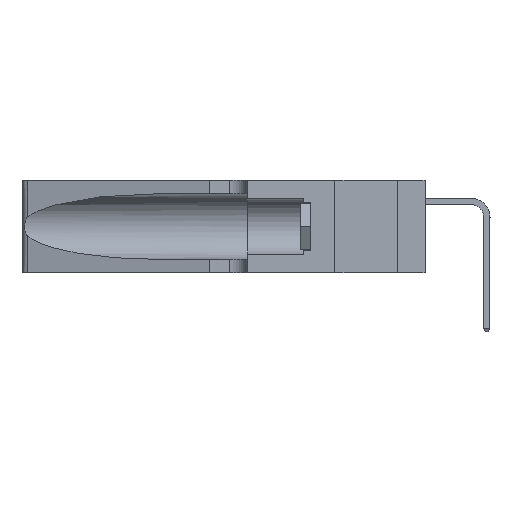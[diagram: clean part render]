
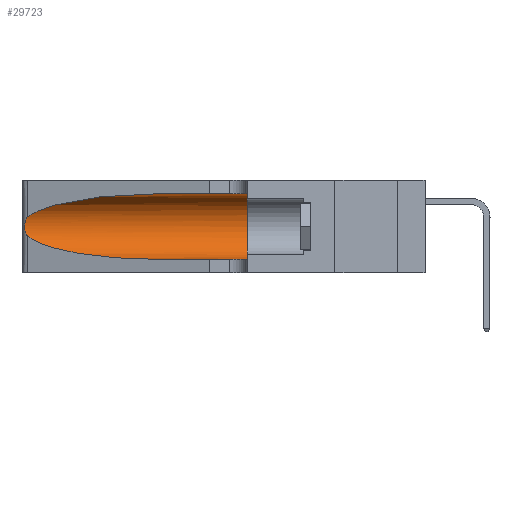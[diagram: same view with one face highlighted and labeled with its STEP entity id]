
A CAD part, left-side view. The second image highlights one B-rep face of the part: STEP entity #29723.
In plain terms, the highlighted cylindrical face has radius 3.308 mm (diameter 6.617 mm), a partial arc.
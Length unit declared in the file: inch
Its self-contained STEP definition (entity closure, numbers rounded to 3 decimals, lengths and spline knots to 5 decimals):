
#167 = ORIENTED_EDGE ( 'NONE', *, *, #20229, .T. ) ;
#437 = AXIS2_PLACEMENT_3D ( 'NONE', #23737, #39651, #20518 ) ;
#1509 = CARTESIAN_POINT ( 'NONE',  ( 0.25487, 1.22718, 0.22369 ) ) ;
#1642 = CARTESIAN_POINT ( 'NONE',  ( 0.25856, 1.23593, 0.16098 ) ) ;
#2059 = VERTEX_POINT ( 'NONE', #39702 ) ;
#2282 = VERTEX_POINT ( 'NONE', #24754 ) ;
#3160 = ORIENTED_EDGE ( 'NONE', *, *, #30647, .F. ) ;
#4863 = CARTESIAN_POINT ( 'NONE',  ( 0.25639, 1.23186, 0.15144 ) ) ;
#5967 = CARTESIAN_POINT ( 'NONE',  ( 0.18966, 0.96281, 0.31525 ) ) ;
#6445 = CARTESIAN_POINT ( 'NONE',  ( 0.25487, 1.22718, 0.14631 ) ) ;
#8058 = CARTESIAN_POINT ( 'NONE',  ( 0.25487, 1.22718, 0.14631 ) ) ;
#9328 = LINE ( 'NONE', #19906, #35790 ) ;
#9596 = CARTESIAN_POINT ( 'NONE',  ( 0.1305, 0.35, 0.05475 ) ) ;
#10426 = CYLINDRICAL_SURFACE ( 'NONE', #437, 0.13025 ) ;
#11134 = CARTESIAN_POINT ( 'NONE',  ( 0.25639, 1.23184, 0.21858 ) ) ;
#11966 = EDGE_CURVE ( 'NONE', #2282, #15474, #9328, .T. ) ;
#12347 = CARTESIAN_POINT ( 'NONE',  ( 0.1305, 1.61858, 0.31525 ) ) ;
#14373 = CARTESIAN_POINT ( 'NONE',  ( 0.25854, 1.2359, 0.20912 ) ) ;
#14772 = CARTESIAN_POINT ( 'NONE',  ( 0.1305, 0.35, 0.185 ) ) ;
#15474 = VERTEX_POINT ( 'NONE', #9596 ) ;
#15602 = CARTESIAN_POINT ( 'NONE',  ( 0.1305, 0.72297, 0.31525 ) ) ;
#15966 = AXIS2_PLACEMENT_3D ( 'NONE', #14772, #37096, #17969 ) ;
#16112 = CARTESIAN_POINT ( 'NONE',  ( 0.2373, 1.15595, 0.08982 ) ) ;
#16342 = CARTESIAN_POINT ( 'NONE',  ( 0.1305, 0.72297, 0.31525 ) ) ;
#16795 = VERTEX_POINT ( 'NONE', #16342 ) ;
#17569 = CARTESIAN_POINT ( 'NONE',  ( 0.26075, 1.23896, 0.19203 ) ) ;
#17969 = DIRECTION ( 'NONE',  ( 0., 0., 1. ) ) ;
#18198 =( BOUNDED_CURVE ( )  B_SPLINE_CURVE ( 3, ( #35230, #16112, #38451, #19336 ),
 .UNSPECIFIED., .F., .F. ) 
 B_SPLINE_CURVE_WITH_KNOTS ( ( 4, 4 ),
 ( 3.44316, 4.71239 ),
 .UNSPECIFIED. ) 
 CURVE ( )  GEOMETRIC_REPRESENTATION_ITEM ( )  RATIONAL_B_SPLINE_CURVE ( ( 1., 0.87, 0.87, 1. ) ) 
 REPRESENTATION_ITEM ( '' )  );
#18345 = VERTEX_POINT ( 'NONE', #6445 ) ;
#18705 = ORIENTED_EDGE ( 'NONE', *, *, #19258, .F. ) ;
#18824 = CARTESIAN_POINT ( 'NONE',  ( 0.2373, 1.15595, 0.28018 ) ) ;
#19258 = EDGE_CURVE ( 'NONE', #2059, #15474, #34302, .T. ) ;
#19336 = CARTESIAN_POINT ( 'NONE',  ( 0.1305, 0.72297, 0.05475 ) ) ;
#19906 = CARTESIAN_POINT ( 'NONE',  ( 0.1305, 1.61858, 0.05475 ) ) ;
#20229 = EDGE_CURVE ( 'NONE', #24245, #18345, #38668, .T. ) ;
#20293 = EDGE_LOOP ( 'NONE', ( #31163, #167, #30415, #21150, #18705, #3160 ) ) ;
#20518 = DIRECTION ( 'NONE',  ( 0., 0., -1. ) ) ;
#20784 = CARTESIAN_POINT ( 'NONE',  ( 0.26017, 1.23833, 0.17102 ) ) ;
#21100 = EDGE_CURVE ( 'NONE', #18345, #2282, #18198, .T. ) ;
#21150 = ORIENTED_EDGE ( 'NONE', *, *, #11966, .T. ) ;
#23116 = DIRECTION ( 'NONE',  ( 0., -1., 0. ) ) ;
#23737 = CARTESIAN_POINT ( 'NONE',  ( 0.1305, 1.61858, 0.185 ) ) ;
#24008 = CARTESIAN_POINT ( 'NONE',  ( 0.25789, 1.23486, 0.15765 ) ) ;
#24245 = VERTEX_POINT ( 'NONE', #39975 ) ;
#24754 = CARTESIAN_POINT ( 'NONE',  ( 0.1305, 0.72297, 0.05475 ) ) ;
#25411 =( BOUNDED_CURVE ( )  B_SPLINE_CURVE ( 3, ( #15602, #5967, #18824, #41153 ),
 .UNSPECIFIED., .F., .T. ) 
 B_SPLINE_CURVE_WITH_KNOTS ( ( 4, 4 ),
 ( 1.5708, 2.84003 ),
 .UNSPECIFIED. ) 
 CURVE ( )  GEOMETRIC_REPRESENTATION_ITEM ( )  RATIONAL_B_SPLINE_CURVE ( ( 1., 0.87, 0.87, 1. ) ) 
 REPRESENTATION_ITEM ( '' )  );
#27078 = CARTESIAN_POINT ( 'NONE',  ( 0.25555, 1.22994, 0.2215 ) ) ;
#27213 = CARTESIAN_POINT ( 'NONE',  ( 0.25555, 1.22993, 0.14849 ) ) ;
#27565 = EDGE_CURVE ( 'NONE', #16795, #24245, #25411, .T. ) ;
#29723 = ADVANCED_FACE ( 'NONE', ( #35887 ), #10426, .F. ) ;
#30415 = ORIENTED_EDGE ( 'NONE', *, *, #21100, .T. ) ;
#30647 = EDGE_CURVE ( 'NONE', #16795, #2059, #40603, .T. ) ;
#31163 = ORIENTED_EDGE ( 'NONE', *, *, #27565, .T. ) ;
#33114 = VECTOR ( 'NONE', #34684, 39.37008 ) ;
#33478 = CARTESIAN_POINT ( 'NONE',  ( 0.25787, 1.23484, 0.2124 ) ) ;
#34302 = CIRCLE ( 'NONE', #15966, 0.13025 ) ;
#34684 = DIRECTION ( 'NONE',  ( 0., -1., 0. ) ) ;
#35230 = CARTESIAN_POINT ( 'NONE',  ( 0.25487, 1.22718, 0.14631 ) ) ;
#35790 = VECTOR ( 'NONE', #23116, 39.37008 ) ;
#35887 = FACE_OUTER_BOUND ( 'NONE', #20293, .T. ) ;
#36676 = CARTESIAN_POINT ( 'NONE',  ( 0.26018, 1.23835, 0.19895 ) ) ;
#37096 = DIRECTION ( 'NONE',  ( 0., 1., 0. ) ) ;
#38451 = CARTESIAN_POINT ( 'NONE',  ( 0.18966, 0.96281, 0.05475 ) ) ;
#38668 = B_SPLINE_CURVE_WITH_KNOTS ( 'NONE', 3,
 ( #1509, #27078, #11134, #33478, #14373, #36676, #17569, #39915, #20784, #1642, #24008, #4863, #27213, #8058 ),
 .UNSPECIFIED., .F., .F.,
 ( 4, 2, 2, 2, 2, 2, 4 ),
 ( 0., 0.00027, 0.00053, 0.00107, 0.0016, 0.00187, 0.00214 ),
 .UNSPECIFIED. ) ;
#39651 = DIRECTION ( 'NONE',  ( 0., -1., 0. ) ) ;
#39702 = CARTESIAN_POINT ( 'NONE',  ( 0.1305, 0.35, 0.31525 ) ) ;
#39915 = CARTESIAN_POINT ( 'NONE',  ( 0.26075, 1.23896, 0.178 ) ) ;
#39975 = CARTESIAN_POINT ( 'NONE',  ( 0.25487, 1.22718, 0.22369 ) ) ;
#40603 = LINE ( 'NONE', #12347, #33114 ) ;
#41153 = CARTESIAN_POINT ( 'NONE',  ( 0.25487, 1.22718, 0.22369 ) ) ;
